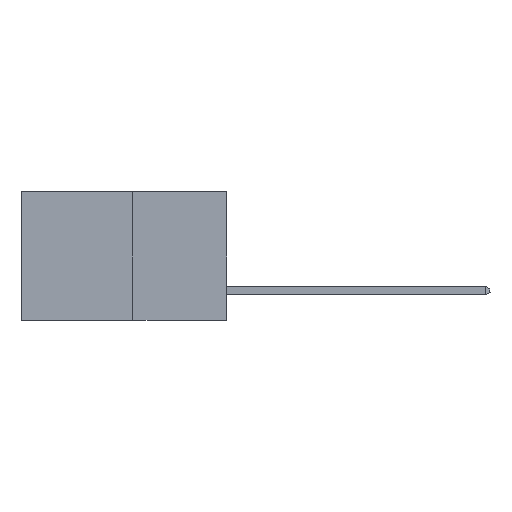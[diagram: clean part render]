
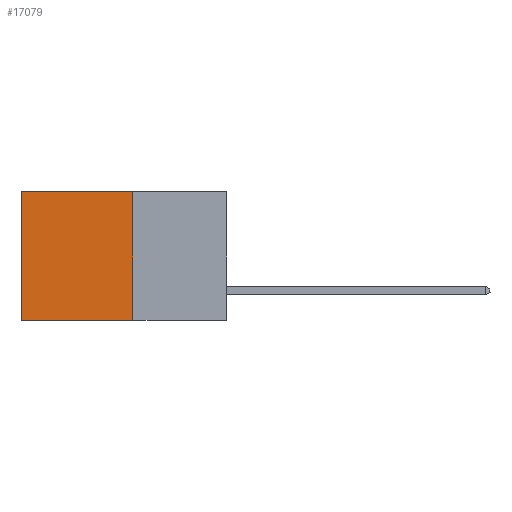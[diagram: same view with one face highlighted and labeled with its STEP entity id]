
A CAD part, left-side view. The second image highlights one B-rep face of the part: STEP entity #17079.
In plain terms, the highlighted planar face has unit normal (-1, 0, 0).
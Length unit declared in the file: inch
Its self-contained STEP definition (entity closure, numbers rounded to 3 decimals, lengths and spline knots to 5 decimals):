
#97 = DIRECTION ( 'NONE',  ( 1., 0., 0. ) ) ;
#318 = VERTEX_POINT ( 'NONE', #8769 ) ;
#370 = CARTESIAN_POINT ( 'NONE',  ( 0.277, 0.27, -0.37 ) ) ;
#617 = VECTOR ( 'NONE', #13395, 39.37008 ) ;
#900 = ORIENTED_EDGE ( 'NONE', *, *, #13900, .F. ) ;
#2231 = DIRECTION ( 'NONE',  ( 0., 1., 0. ) ) ;
#3706 = LINE ( 'NONE', #10577, #13467 ) ;
#4333 = LINE ( 'NONE', #12035, #617 ) ;
#5528 = ORIENTED_EDGE ( 'NONE', *, *, #17586, .T. ) ;
#6502 = CARTESIAN_POINT ( 'NONE',  ( 0.277, 0.27, -0.37 ) ) ;
#6873 = LINE ( 'NONE', #6502, #17412 ) ;
#7980 = EDGE_LOOP ( 'NONE', ( #5528, #14735, #900, #17390 ) ) ;
#8353 = CARTESIAN_POINT ( 'NONE',  ( 0.277, 0.59, -0.37 ) ) ;
#8769 = CARTESIAN_POINT ( 'NONE',  ( 0.277, 0.59, 0. ) ) ;
#9791 = DIRECTION ( 'NONE',  ( 0., 0., -1. ) ) ;
#9863 = DIRECTION ( 'NONE',  ( 0., 0., -1. ) ) ;
#10577 = CARTESIAN_POINT ( 'NONE',  ( 0.277, 0.27, -0.37 ) ) ;
#11892 = VECTOR ( 'NONE', #9791, 39.37008 ) ;
#12035 = CARTESIAN_POINT ( 'NONE',  ( 0.277, 0.27, 0. ) ) ;
#12073 = EDGE_CURVE ( 'NONE', #12503, #13693, #3706, .T. ) ;
#12132 = DIRECTION ( 'NONE',  ( 0., 0., -1. ) ) ;
#12408 = VERTEX_POINT ( 'NONE', #12677 ) ;
#12503 = VERTEX_POINT ( 'NONE', #370 ) ;
#12677 = CARTESIAN_POINT ( 'NONE',  ( 0.277, 0.27, 0. ) ) ;
#13157 = EDGE_CURVE ( 'NONE', #12408, #318, #4333, .T. ) ;
#13395 = DIRECTION ( 'NONE',  ( 0., 1., 0. ) ) ;
#13467 = VECTOR ( 'NONE', #2231, 39.37008 ) ;
#13693 = VERTEX_POINT ( 'NONE', #17068 ) ;
#13900 = EDGE_CURVE ( 'NONE', #12408, #12503, #6873, .T. ) ;
#13951 = CARTESIAN_POINT ( 'NONE',  ( 0.277, 0.27, -0.37 ) ) ;
#14735 = ORIENTED_EDGE ( 'NONE', *, *, #12073, .F. ) ;
#15874 = LINE ( 'NONE', #8353, #11892 ) ;
#16624 = PLANE ( 'NONE',  #17466 ) ;
#16718 = FACE_OUTER_BOUND ( 'NONE', #7980, .T. ) ;
#17068 = CARTESIAN_POINT ( 'NONE',  ( 0.277, 0.59, -0.37 ) ) ;
#17079 = ADVANCED_FACE ( 'NONE', ( #16718 ), #16624, .F. ) ;
#17390 = ORIENTED_EDGE ( 'NONE', *, *, #13157, .T. ) ;
#17412 = VECTOR ( 'NONE', #12132, 39.37008 ) ;
#17466 = AXIS2_PLACEMENT_3D ( 'NONE', #13951, #97, #9863 ) ;
#17586 = EDGE_CURVE ( 'NONE', #318, #13693, #15874, .T. ) ;
